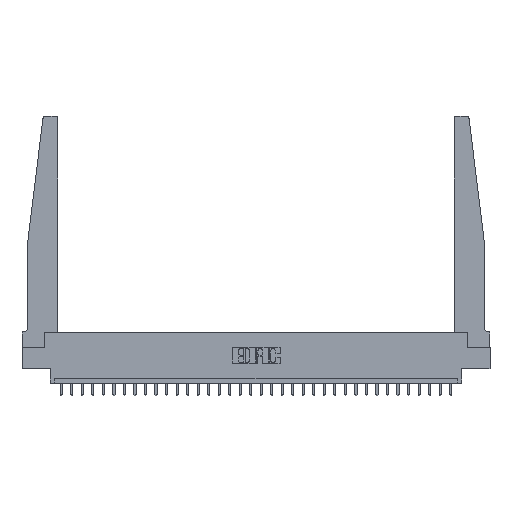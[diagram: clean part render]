
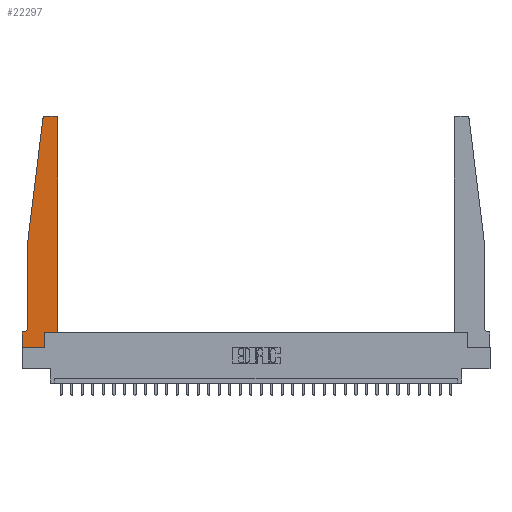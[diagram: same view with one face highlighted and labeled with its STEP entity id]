
A CAD part, top view. The second image highlights one B-rep face of the part: STEP entity #22297.
In plain terms, the highlighted planar face has unit normal (0, 0, 1).
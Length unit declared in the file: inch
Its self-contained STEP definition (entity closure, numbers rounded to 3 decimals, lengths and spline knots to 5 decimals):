
#238 = CARTESIAN_POINT ( 'NONE',  ( 0.425, 0.18, 0.37 ) ) ;
#452 = FACE_OUTER_BOUND ( 'NONE', #19080, .T. ) ;
#463 = CARTESIAN_POINT ( 'NONE',  ( 0.425, 0.18, 0.37 ) ) ;
#651 = DIRECTION ( 'NONE',  ( 0., 0., -1. ) ) ;
#718 = VERTEX_POINT ( 'NONE', #4834 ) ;
#1458 = CARTESIAN_POINT ( 'NONE',  ( 0.395, 2.75, 0.37 ) ) ;
#1478 = DIRECTION ( 'NONE',  ( 1., 0., 0. ) ) ;
#1585 = EDGE_CURVE ( 'NONE', #21965, #6192, #3207, .T. ) ;
#1706 = DIRECTION ( 'NONE',  ( -0.122, -0.992, 0. ) ) ;
#2133 = ORIENTED_EDGE ( 'NONE', *, *, #3651, .T. ) ;
#2523 = CARTESIAN_POINT ( 'NONE',  ( 0., 0.1875, 0.37 ) ) ;
#3207 = LINE ( 'NONE', #10382, #12309 ) ;
#3651 = EDGE_CURVE ( 'NONE', #10240, #8331, #19933, .T. ) ;
#3839 = VECTOR ( 'NONE', #28363, 39.37008 ) ;
#4245 = LINE ( 'NONE', #19819, #27374 ) ;
#4346 = VERTEX_POINT ( 'NONE', #7583 ) ;
#4583 = DIRECTION ( 'NONE',  ( 0., 0., 1. ) ) ;
#4698 = LINE ( 'NONE', #16291, #14477 ) ;
#4834 = CARTESIAN_POINT ( 'NONE',  ( 0.425, 2.72, 0.37 ) ) ;
#5154 = CARTESIAN_POINT ( 'NONE',  ( 0.015, 0.2375, 0.37 ) ) ;
#5341 = DIRECTION ( 'NONE',  ( -1., 0., 0. ) ) ;
#5639 = LINE ( 'NONE', #463, #19281 ) ;
#6035 = ORIENTED_EDGE ( 'NONE', *, *, #1585, .T. ) ;
#6192 = VERTEX_POINT ( 'NONE', #24350 ) ;
#6221 = EDGE_CURVE ( 'NONE', #8331, #12793, #21517, .T. ) ;
#6682 = CARTESIAN_POINT ( 'NONE',  ( 0.065, 0.2375, 0.37 ) ) ;
#6881 = CARTESIAN_POINT ( 'NONE',  ( 0.015, 0.1875, 0.37 ) ) ;
#7135 = ORIENTED_EDGE ( 'NONE', *, *, #9241, .T. ) ;
#7274 = PLANE ( 'NONE',  #27771 ) ;
#7583 = CARTESIAN_POINT ( 'NONE',  ( 0.2605, 0.18, 0.37 ) ) ;
#7637 = ORIENTED_EDGE ( 'NONE', *, *, #17159, .T. ) ;
#8084 = CARTESIAN_POINT ( 'NONE',  ( 0.395, 2.72, 0.37 ) ) ;
#8331 = VERTEX_POINT ( 'NONE', #13631 ) ;
#8678 = EDGE_CURVE ( 'NONE', #10994, #21965, #9071, .T. ) ;
#9071 = LINE ( 'NONE', #12500, #3839 ) ;
#9241 = EDGE_CURVE ( 'NONE', #6192, #4346, #16746, .T. ) ;
#10195 = DIRECTION ( 'NONE',  ( 0., 1., 0. ) ) ;
#10240 = VERTEX_POINT ( 'NONE', #12403 ) ;
#10382 = CARTESIAN_POINT ( 'NONE',  ( 0., 0., 0.37 ) ) ;
#10994 = VERTEX_POINT ( 'NONE', #22984 ) ;
#12309 = VECTOR ( 'NONE', #1478, 39.37008 ) ;
#12403 = CARTESIAN_POINT ( 'NONE',  ( 0.27653, 2.75, 0.37 ) ) ;
#12412 = DIRECTION ( 'NONE',  ( -1., 0., 0. ) ) ;
#12500 = CARTESIAN_POINT ( 'NONE',  ( 0., 0., 0.37 ) ) ;
#12793 = VERTEX_POINT ( 'NONE', #27729 ) ;
#12987 = VECTOR ( 'NONE', #22471, 39.37008 ) ;
#13631 = CARTESIAN_POINT ( 'NONE',  ( 0.24675, 2.72367, 0.37 ) ) ;
#13941 = DIRECTION ( 'NONE',  ( 0., 0., 1. ) ) ;
#14477 = VECTOR ( 'NONE', #5341, 39.37008 ) ;
#14745 = AXIS2_PLACEMENT_3D ( 'NONE', #5154, #651, #22980 ) ;
#14786 = AXIS2_PLACEMENT_3D ( 'NONE', #8084, #24085, #17864 ) ;
#14994 = ORIENTED_EDGE ( 'NONE', *, *, #17433, .T. ) ;
#15437 = CARTESIAN_POINT ( 'NONE',  ( 0.27653, 2.72, 0.37 ) ) ;
#15976 = DIRECTION ( 'NONE',  ( 1., 0., 0. ) ) ;
#16291 = CARTESIAN_POINT ( 'NONE',  ( 0.065, 0.1875, 0.37 ) ) ;
#16736 = ORIENTED_EDGE ( 'NONE', *, *, #28079, .T. ) ;
#16746 = LINE ( 'NONE', #23664, #27987 ) ;
#17155 = EDGE_CURVE ( 'NONE', #20917, #22744, #18576, .T. ) ;
#17159 = EDGE_CURVE ( 'NONE', #19374, #718, #5639, .T. ) ;
#17337 = EDGE_CURVE ( 'NONE', #12793, #20917, #4245, .T. ) ;
#17433 = EDGE_CURVE ( 'NONE', #4346, #19374, #23501, .T. ) ;
#17531 = CARTESIAN_POINT ( 'NONE',  ( 0.065, 1.25, 0.37 ) ) ;
#17598 = CIRCLE ( 'NONE', #14786, 0.03 ) ;
#17864 = DIRECTION ( 'NONE',  ( 1., 0., 0. ) ) ;
#18448 = VERTEX_POINT ( 'NONE', #1458 ) ;
#18576 = CIRCLE ( 'NONE', #14745, 0.05 ) ;
#19080 = EDGE_LOOP ( 'NONE', ( #16736, #2133, #28054, #23286, #27029, #19213, #27974, #6035, #7135, #14994, #7637, #27281 ) ) ;
#19213 = ORIENTED_EDGE ( 'NONE', *, *, #21693, .T. ) ;
#19281 = VECTOR ( 'NONE', #25235, 39.37008 ) ;
#19374 = VERTEX_POINT ( 'NONE', #238 ) ;
#19819 = CARTESIAN_POINT ( 'NONE',  ( 0.065, 1.25, 0.37 ) ) ;
#19933 = CIRCLE ( 'NONE', #20728, 0.03 ) ;
#20728 = AXIS2_PLACEMENT_3D ( 'NONE', #15437, #4583, #22501 ) ;
#20917 = VERTEX_POINT ( 'NONE', #6682 ) ;
#21414 = CARTESIAN_POINT ( 'NONE',  ( 0.25, 2.75, 0.37 ) ) ;
#21517 = LINE ( 'NONE', #17531, #21878 ) ;
#21693 = EDGE_CURVE ( 'NONE', #22744, #10994, #4698, .T. ) ;
#21878 = VECTOR ( 'NONE', #1706, 39.37008 ) ;
#21965 = VERTEX_POINT ( 'NONE', #28288 ) ;
#22171 = DIRECTION ( 'NONE',  ( 0., -1., 0. ) ) ;
#22297 = ADVANCED_FACE ( 'NONE', ( #452 ), #7274, .T. ) ;
#22471 = DIRECTION ( 'NONE',  ( 1., 0., 0. ) ) ;
#22501 = DIRECTION ( 'NONE',  ( 1., 0., 0. ) ) ;
#22744 = VERTEX_POINT ( 'NONE', #6881 ) ;
#22980 = DIRECTION ( 'NONE',  ( -1., 0., 0. ) ) ;
#22984 = CARTESIAN_POINT ( 'NONE',  ( 0., 0.1875, 0.37 ) ) ;
#23066 = EDGE_CURVE ( 'NONE', #718, #18448, #17598, .T. ) ;
#23286 = ORIENTED_EDGE ( 'NONE', *, *, #17337, .T. ) ;
#23501 = LINE ( 'NONE', #27063, #12987 ) ;
#23664 = CARTESIAN_POINT ( 'NONE',  ( 0.2605, 0.18, 0.37 ) ) ;
#24085 = DIRECTION ( 'NONE',  ( 0., 0., 1. ) ) ;
#24350 = CARTESIAN_POINT ( 'NONE',  ( 0.2605, 0., 0.37 ) ) ;
#25235 = DIRECTION ( 'NONE',  ( 0., 1., 0. ) ) ;
#25710 = VECTOR ( 'NONE', #12412, 39.37008 ) ;
#26778 = LINE ( 'NONE', #21414, #25710 ) ;
#27029 = ORIENTED_EDGE ( 'NONE', *, *, #17155, .T. ) ;
#27063 = CARTESIAN_POINT ( 'NONE',  ( 0.425, 0.18, 0.37 ) ) ;
#27281 = ORIENTED_EDGE ( 'NONE', *, *, #23066, .T. ) ;
#27374 = VECTOR ( 'NONE', #22171, 39.37008 ) ;
#27729 = CARTESIAN_POINT ( 'NONE',  ( 0.065, 1.25, 0.37 ) ) ;
#27771 = AXIS2_PLACEMENT_3D ( 'NONE', #2523, #13941, #15976 ) ;
#27974 = ORIENTED_EDGE ( 'NONE', *, *, #8678, .T. ) ;
#27987 = VECTOR ( 'NONE', #10195, 39.37008 ) ;
#28054 = ORIENTED_EDGE ( 'NONE', *, *, #6221, .T. ) ;
#28079 = EDGE_CURVE ( 'NONE', #18448, #10240, #26778, .T. ) ;
#28288 = CARTESIAN_POINT ( 'NONE',  ( 0., 0., 0.37 ) ) ;
#28363 = DIRECTION ( 'NONE',  ( 0., -1., 0. ) ) ;
